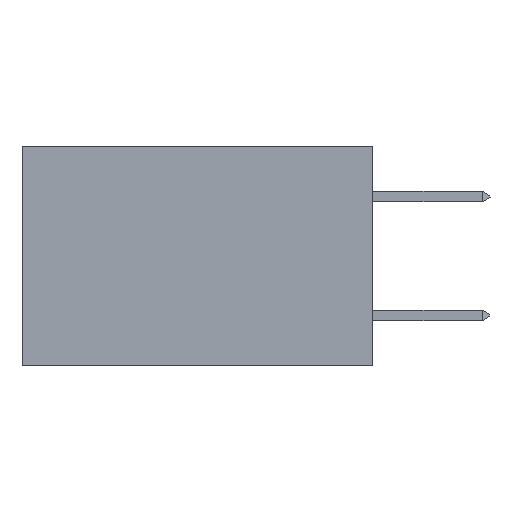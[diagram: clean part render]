
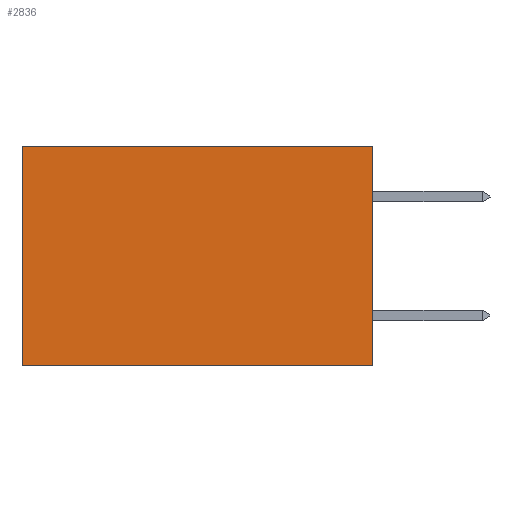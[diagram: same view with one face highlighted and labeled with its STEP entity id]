
A CAD part, left-side view. The second image highlights one B-rep face of the part: STEP entity #2836.
In plain terms, the highlighted planar face has unit normal (-1, 0, 0).
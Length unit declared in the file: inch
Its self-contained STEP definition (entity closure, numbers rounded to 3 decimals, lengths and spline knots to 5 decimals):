
#337 = CARTESIAN_POINT ( 'NONE',  ( 0.277, 0.59, -0.37 ) ) ;
#563 = DIRECTION ( 'NONE',  ( 0., 1., 0. ) ) ;
#571 = CARTESIAN_POINT ( 'NONE',  ( 0.277, 0., 0. ) ) ;
#731 = CARTESIAN_POINT ( 'NONE',  ( 0.277, 0., 0. ) ) ;
#921 = CARTESIAN_POINT ( 'NONE',  ( 0.277, 0., -0.37 ) ) ;
#940 = LINE ( 'NONE', #571, #7507 ) ;
#1080 = DIRECTION ( 'NONE',  ( 0., 0., -1. ) ) ;
#1957 = DIRECTION ( 'NONE',  ( 0., 0., -1. ) ) ;
#2080 = VECTOR ( 'NONE', #5421, 39.37008 ) ;
#2193 = CARTESIAN_POINT ( 'NONE',  ( 0.277, 0., -0.37 ) ) ;
#2400 = VECTOR ( 'NONE', #1957, 39.37008 ) ;
#2470 = DIRECTION ( 'NONE',  ( 0., 0., -1. ) ) ;
#2836 = ADVANCED_FACE ( 'NONE', ( #3871 ), #5671, .F. ) ;
#2856 = VERTEX_POINT ( 'NONE', #6732 ) ;
#3019 = EDGE_CURVE ( 'NONE', #2856, #6139, #7796, .T. ) ;
#3155 = VERTEX_POINT ( 'NONE', #7425 ) ;
#3320 = EDGE_CURVE ( 'NONE', #5505, #3155, #6088, .T. ) ;
#3372 = CARTESIAN_POINT ( 'NONE',  ( 0.277, 0.59, -0.37 ) ) ;
#3743 = LINE ( 'NONE', #921, #2080 ) ;
#3871 = FACE_OUTER_BOUND ( 'NONE', #7962, .T. ) ;
#4385 = CARTESIAN_POINT ( 'NONE',  ( 0.277, 0., -0.37 ) ) ;
#4498 = ORIENTED_EDGE ( 'NONE', *, *, #3019, .T. ) ;
#4513 = ORIENTED_EDGE ( 'NONE', *, *, #7629, .F. ) ;
#4524 = ORIENTED_EDGE ( 'NONE', *, *, #3320, .F. ) ;
#4541 = ORIENTED_EDGE ( 'NONE', *, *, #6493, .T. ) ;
#5421 = DIRECTION ( 'NONE',  ( 0., 1., 0. ) ) ;
#5505 = VERTEX_POINT ( 'NONE', #731 ) ;
#5671 = PLANE ( 'NONE',  #7103 ) ;
#5985 = VECTOR ( 'NONE', #1080, 39.37008 ) ;
#6088 = LINE ( 'NONE', #2193, #2400 ) ;
#6139 = VERTEX_POINT ( 'NONE', #3372 ) ;
#6493 = EDGE_CURVE ( 'NONE', #5505, #2856, #940, .T. ) ;
#6600 = DIRECTION ( 'NONE',  ( 1., 0., 0. ) ) ;
#6732 = CARTESIAN_POINT ( 'NONE',  ( 0.277, 0.59, 0. ) ) ;
#7103 = AXIS2_PLACEMENT_3D ( 'NONE', #4385, #6600, #2470 ) ;
#7425 = CARTESIAN_POINT ( 'NONE',  ( 0.277, 0., -0.37 ) ) ;
#7507 = VECTOR ( 'NONE', #563, 39.37008 ) ;
#7629 = EDGE_CURVE ( 'NONE', #3155, #6139, #3743, .T. ) ;
#7796 = LINE ( 'NONE', #337, #5985 ) ;
#7962 = EDGE_LOOP ( 'NONE', ( #4498, #4513, #4524, #4541 ) ) ;
